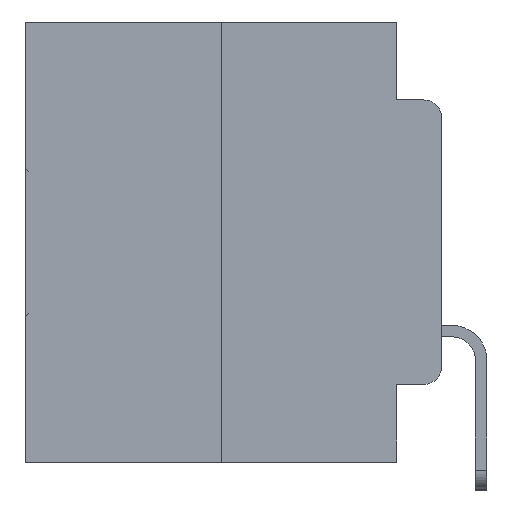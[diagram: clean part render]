
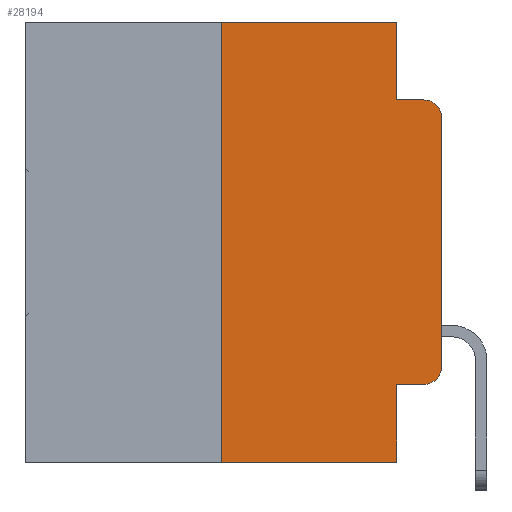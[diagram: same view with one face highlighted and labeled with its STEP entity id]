
A CAD part, left-side view. The second image highlights one B-rep face of the part: STEP entity #28194.
In plain terms, the highlighted planar face has unit normal (-1, 0, 0).
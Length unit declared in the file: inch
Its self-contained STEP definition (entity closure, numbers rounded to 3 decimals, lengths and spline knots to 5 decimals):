
#130 = DIRECTION ( 'NONE',  ( 0., 0., -1. ) ) ;
#176 = VERTEX_POINT ( 'NONE', #20622 ) ;
#211 = CIRCLE ( 'NONE', #7189, 0.02 ) ;
#308 = LINE ( 'NONE', #24072, #12188 ) ;
#500 = ORIENTED_EDGE ( 'NONE', *, *, #16250, .F. ) ;
#863 = VERTEX_POINT ( 'NONE', #29354 ) ;
#898 = DIRECTION ( 'NONE',  ( 0., -1., 0. ) ) ;
#1320 = EDGE_CURVE ( 'NONE', #20943, #6534, #10827, .T. ) ;
#1407 = CARTESIAN_POINT ( 'NONE',  ( 0., 0., 0. ) ) ;
#1958 = AXIS2_PLACEMENT_3D ( 'NONE', #22727, #9091, #24997 ) ;
#2037 = ORIENTED_EDGE ( 'NONE', *, *, #16456, .F. ) ;
#3449 = VERTEX_POINT ( 'NONE', #14037 ) ;
#4465 = CARTESIAN_POINT ( 'NONE',  ( 0., 0., -0.1085 ) ) ;
#4541 = ORIENTED_EDGE ( 'NONE', *, *, #13555, .F. ) ;
#6107 = LINE ( 'NONE', #6482, #11598 ) ;
#6359 = DIRECTION ( 'NONE',  ( 0., 0., -1. ) ) ;
#6482 = CARTESIAN_POINT ( 'NONE',  ( 0., 0.051, 0. ) ) ;
#6534 = VERTEX_POINT ( 'NONE', #19631 ) ;
#6616 = EDGE_LOOP ( 'NONE', ( #12869, #24022, #500, #24738, #13839, #2037, #10881, #4541, #8055, #28340 ) ) ;
#7189 = AXIS2_PLACEMENT_3D ( 'NONE', #27744, #14291, #130 ) ;
#8055 = ORIENTED_EDGE ( 'NONE', *, *, #19447, .T. ) ;
#8438 = AXIS2_PLACEMENT_3D ( 'NONE', #24547, #20122, #6359 ) ;
#8617 = DIRECTION ( 'NONE',  ( 0., 0., 1. ) ) ;
#8666 = VERTEX_POINT ( 'NONE', #20904 ) ;
#9091 = DIRECTION ( 'NONE',  ( -1., 0., 0. ) ) ;
#9252 = EDGE_CURVE ( 'NONE', #8666, #11177, #11247, .T. ) ;
#10827 = LINE ( 'NONE', #13356, #27446 ) ;
#10881 = ORIENTED_EDGE ( 'NONE', *, *, #22057, .T. ) ;
#11177 = VERTEX_POINT ( 'NONE', #12301 ) ;
#11247 = CIRCLE ( 'NONE', #1958, 0.02 ) ;
#11429 = VERTEX_POINT ( 'NONE', #22182 ) ;
#11598 = VECTOR ( 'NONE', #24770, 39.37008 ) ;
#11944 = VECTOR ( 'NONE', #28951, 39.37008 ) ;
#12188 = VECTOR ( 'NONE', #898, 39.37008 ) ;
#12301 = CARTESIAN_POINT ( 'NONE',  ( 0., 0., -0.3915 ) ) ;
#12455 = EDGE_CURVE ( 'NONE', #3449, #20943, #23387, .T. ) ;
#12869 = ORIENTED_EDGE ( 'NONE', *, *, #21447, .T. ) ;
#13254 = VECTOR ( 'NONE', #29280, 39.37008 ) ;
#13356 = CARTESIAN_POINT ( 'NONE',  ( 0., 0.051, 0. ) ) ;
#13555 = EDGE_CURVE ( 'NONE', #176, #15750, #6107, .T. ) ;
#13580 = CARTESIAN_POINT ( 'NONE',  ( 0., 0.25, 0. ) ) ;
#13839 = ORIENTED_EDGE ( 'NONE', *, *, #12455, .F. ) ;
#14037 = CARTESIAN_POINT ( 'NONE',  ( 0., 0.25, 0. ) ) ;
#14291 = DIRECTION ( 'NONE',  ( -1., 0., 0. ) ) ;
#15667 = DIRECTION ( 'NONE',  ( 0., 0., -1. ) ) ;
#15750 = VERTEX_POINT ( 'NONE', #17771 ) ;
#16250 = EDGE_CURVE ( 'NONE', #6534, #11429, #308, .T. ) ;
#16456 = EDGE_CURVE ( 'NONE', #863, #3449, #18560, .T. ) ;
#16980 = LINE ( 'NONE', #1407, #21553 ) ;
#17450 = VECTOR ( 'NONE', #28057, 39.37008 ) ;
#17771 = CARTESIAN_POINT ( 'NONE',  ( 0., 0.051, -0.5 ) ) ;
#18560 = LINE ( 'NONE', #13580, #13254 ) ;
#18607 = DIRECTION ( 'NONE',  ( 0., -1., 0. ) ) ;
#19447 = EDGE_CURVE ( 'NONE', #176, #8666, #23458, .T. ) ;
#19631 = CARTESIAN_POINT ( 'NONE',  ( 0., 0.051, -0.0885 ) ) ;
#20122 = DIRECTION ( 'NONE',  ( 1., 0., 0. ) ) ;
#20622 = CARTESIAN_POINT ( 'NONE',  ( 0., 0.051, -0.4115 ) ) ;
#20904 = CARTESIAN_POINT ( 'NONE',  ( 0., 0.02, -0.4115 ) ) ;
#20943 = VERTEX_POINT ( 'NONE', #22693 ) ;
#21329 = CARTESIAN_POINT ( 'NONE',  ( 0., 0.051, -0.4115 ) ) ;
#21447 = EDGE_CURVE ( 'NONE', #11177, #24165, #16980, .T. ) ;
#21553 = VECTOR ( 'NONE', #8617, 39.37008 ) ;
#22057 = EDGE_CURVE ( 'NONE', #863, #15750, #23987, .T. ) ;
#22182 = CARTESIAN_POINT ( 'NONE',  ( 0., 0.02, -0.0885 ) ) ;
#22652 = VECTOR ( 'NONE', #18607, 39.37008 ) ;
#22693 = CARTESIAN_POINT ( 'NONE',  ( 0., 0.051, 0. ) ) ;
#22727 = CARTESIAN_POINT ( 'NONE',  ( 0., 0.02, -0.3915 ) ) ;
#23163 = CARTESIAN_POINT ( 'NONE',  ( 0., 0.473, 0. ) ) ;
#23387 = LINE ( 'NONE', #23163, #22652 ) ;
#23458 = LINE ( 'NONE', #21329, #17450 ) ;
#23987 = LINE ( 'NONE', #26748, #11944 ) ;
#24022 = ORIENTED_EDGE ( 'NONE', *, *, #24287, .T. ) ;
#24072 = CARTESIAN_POINT ( 'NONE',  ( 0., 0.051, -0.0885 ) ) ;
#24165 = VERTEX_POINT ( 'NONE', #4465 ) ;
#24287 = EDGE_CURVE ( 'NONE', #24165, #11429, #211, .T. ) ;
#24547 = CARTESIAN_POINT ( 'NONE',  ( 0., 0.473, 0. ) ) ;
#24738 = ORIENTED_EDGE ( 'NONE', *, *, #1320, .F. ) ;
#24770 = DIRECTION ( 'NONE',  ( 0., 0., -1. ) ) ;
#24997 = DIRECTION ( 'NONE',  ( 0., 0., -1. ) ) ;
#26748 = CARTESIAN_POINT ( 'NONE',  ( 0., 0.473, -0.5 ) ) ;
#27446 = VECTOR ( 'NONE', #15667, 39.37008 ) ;
#27744 = CARTESIAN_POINT ( 'NONE',  ( 0., 0.02, -0.1085 ) ) ;
#27800 = FACE_OUTER_BOUND ( 'NONE', #6616, .T. ) ;
#28057 = DIRECTION ( 'NONE',  ( 0., -1., 0. ) ) ;
#28194 = ADVANCED_FACE ( 'NONE', ( #27800 ), #28992, .F. ) ;
#28340 = ORIENTED_EDGE ( 'NONE', *, *, #9252, .T. ) ;
#28951 = DIRECTION ( 'NONE',  ( 0., -1., 0. ) ) ;
#28992 = PLANE ( 'NONE',  #8438 ) ;
#29280 = DIRECTION ( 'NONE',  ( 0., 0., 1. ) ) ;
#29354 = CARTESIAN_POINT ( 'NONE',  ( 0., 0.25, -0.5 ) ) ;
